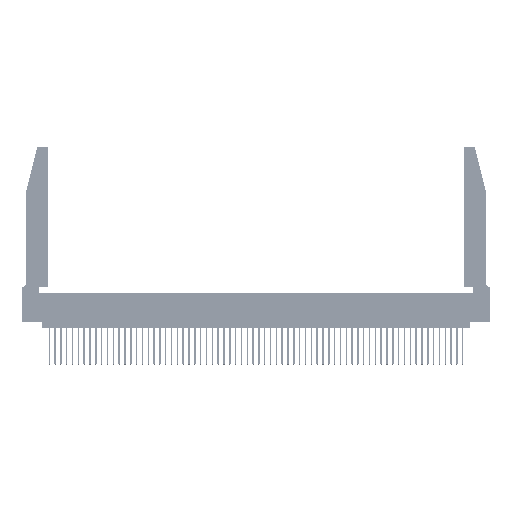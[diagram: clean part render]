
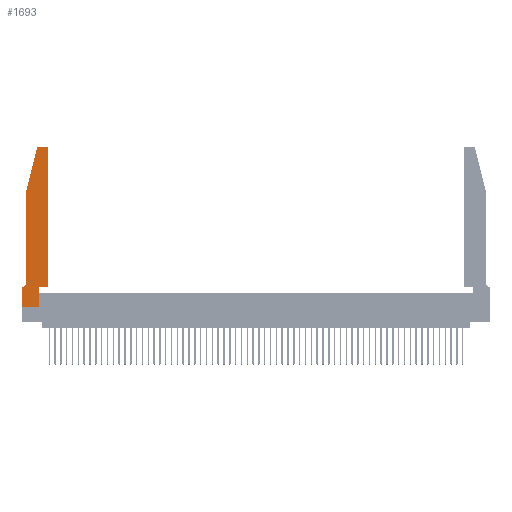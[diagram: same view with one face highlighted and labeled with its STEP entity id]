
A CAD part, top view. The second image highlights one B-rep face of the part: STEP entity #1693.
In plain terms, the highlighted planar face has unit normal (0, 0, 1).
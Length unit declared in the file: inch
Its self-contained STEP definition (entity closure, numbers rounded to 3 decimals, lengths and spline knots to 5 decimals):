
#1656 = CARTESIAN_POINT ( 'NONE',  ( 0.4505, 0.35, 0.37 ) ) ;
#1693 = ADVANCED_FACE ( 'NONE', ( #45413 ), #8325, .T. ) ;
#1998 = ORIENTED_EDGE ( 'NONE', *, *, #39850, .T. ) ;
#2313 = DIRECTION ( 'NONE',  ( -1., 0., 0. ) ) ;
#2681 = VERTEX_POINT ( 'NONE', #39917 ) ;
#3382 = DIRECTION ( 'NONE',  ( 0., 0., 1. ) ) ;
#3571 = EDGE_CURVE ( 'NONE', #25130, #55235, #18703, .T. ) ;
#3941 = LINE ( 'NONE', #18616, #14277 ) ;
#5013 = DIRECTION ( 'NONE',  ( 0., -1., 0. ) ) ;
#5835 = VECTOR ( 'NONE', #31532, 39.37008 ) ;
#6038 = VECTOR ( 'NONE', #40853, 39.37008 ) ;
#6078 = ORIENTED_EDGE ( 'NONE', *, *, #38653, .T. ) ;
#8318 = VERTEX_POINT ( 'NONE', #18544 ) ;
#8325 = PLANE ( 'NONE',  #57042 ) ;
#9174 = CARTESIAN_POINT ( 'NONE',  ( 0.0755, 0.42, 0.37 ) ) ;
#10579 = AXIS2_PLACEMENT_3D ( 'NONE', #34514, #3382, #38793 ) ;
#10895 = DIRECTION ( 'NONE',  ( 1., 0., 0. ) ) ;
#11281 = CARTESIAN_POINT ( 'NONE',  ( 0.284, 2.75, 0.37 ) ) ;
#11627 = LINE ( 'NONE', #30556, #20619 ) ;
#12865 = LINE ( 'NONE', #41238, #6038 ) ;
#14277 = VECTOR ( 'NONE', #27912, 39.37008 ) ;
#16488 = ORIENTED_EDGE ( 'NONE', *, *, #51522, .T. ) ;
#16531 = VERTEX_POINT ( 'NONE', #9174 ) ;
#17021 = CARTESIAN_POINT ( 'NONE',  ( 0., 0.35, 0.37 ) ) ;
#17188 = ORIENTED_EDGE ( 'NONE', *, *, #3571, .T. ) ;
#17287 = VERTEX_POINT ( 'NONE', #27896 ) ;
#17335 = CARTESIAN_POINT ( 'NONE',  ( 0., 0., 0.37 ) ) ;
#18544 = CARTESIAN_POINT ( 'NONE',  ( 0., 0.35, 0.37 ) ) ;
#18616 = CARTESIAN_POINT ( 'NONE',  ( 0.2865, 0.35, 0.37 ) ) ;
#18703 = CIRCLE ( 'NONE', #56364, 0.03 ) ;
#20619 = VECTOR ( 'NONE', #39122, 39.37008 ) ;
#22130 = VERTEX_POINT ( 'NONE', #38931 ) ;
#22216 = CARTESIAN_POINT ( 'NONE',  ( 0.4505, 0.35, 0.37 ) ) ;
#22503 = DIRECTION ( 'NONE',  ( -1., 0., 0. ) ) ;
#23023 = VERTEX_POINT ( 'NONE', #17335 ) ;
#23167 = CARTESIAN_POINT ( 'NONE',  ( 0.0755, 2., 0.37 ) ) ;
#23228 = CARTESIAN_POINT ( 'NONE',  ( 0.25487, 2.72718, 0.37 ) ) ;
#23265 = ORIENTED_EDGE ( 'NONE', *, *, #55868, .T. ) ;
#23733 = LINE ( 'NONE', #31285, #51468 ) ;
#24746 = CARTESIAN_POINT ( 'NONE',  ( 0.0055, 0.35, 0.37 ) ) ;
#24871 = CARTESIAN_POINT ( 'NONE',  ( 0.4505, 0.35, 0.37 ) ) ;
#25130 = VERTEX_POINT ( 'NONE', #11281 ) ;
#25391 = CIRCLE ( 'NONE', #10579, 0.03 ) ;
#26626 = DIRECTION ( 'NONE',  ( 0., -1., 0. ) ) ;
#26824 = CARTESIAN_POINT ( 'NONE',  ( 0., 0., 0.37 ) ) ;
#27221 = LINE ( 'NONE', #53321, #5835 ) ;
#27896 = CARTESIAN_POINT ( 'NONE',  ( 0.2865, 0.35, 0.37 ) ) ;
#27912 = DIRECTION ( 'NONE',  ( 0., 1., 0. ) ) ;
#27951 = EDGE_CURVE ( 'NONE', #49657, #16531, #23733, .T. ) ;
#28055 = CARTESIAN_POINT ( 'NONE',  ( 0.2865, 0., 0.37 ) ) ;
#29270 = EDGE_LOOP ( 'NONE', ( #23265, #17188, #54557, #50282, #1998, #47349, #16488, #56814, #45931, #6078, #56794, #52931 ) ) ;
#29696 = VERTEX_POINT ( 'NONE', #22216 ) ;
#30556 = CARTESIAN_POINT ( 'NONE',  ( 0.0755, 2., 0.37 ) ) ;
#31285 = CARTESIAN_POINT ( 'NONE',  ( 0.0755, 2., 0.37 ) ) ;
#31532 = DIRECTION ( 'NONE',  ( 1., 0., 0. ) ) ;
#31607 = CARTESIAN_POINT ( 'NONE',  ( 0.0755, 0.35, 0.37 ) ) ;
#32679 = CIRCLE ( 'NONE', #56281, 0.07 ) ;
#34514 = CARTESIAN_POINT ( 'NONE',  ( 0.4205, 2.72, 0.37 ) ) ;
#35777 = EDGE_CURVE ( 'NONE', #55235, #49657, #11627, .T. ) ;
#36547 = LINE ( 'NONE', #26824, #56707 ) ;
#36707 = EDGE_CURVE ( 'NONE', #39208, #17287, #3941, .T. ) ;
#37719 = VECTOR ( 'NONE', #10895, 39.37008 ) ;
#37913 = DIRECTION ( 'NONE',  ( 0., 0., -1. ) ) ;
#38653 = EDGE_CURVE ( 'NONE', #17287, #29696, #52315, .T. ) ;
#38656 = DIRECTION ( 'NONE',  ( 1., 0., 0. ) ) ;
#38793 = DIRECTION ( 'NONE',  ( 1., 0., 0. ) ) ;
#38931 = CARTESIAN_POINT ( 'NONE',  ( 0.4505, 2.72, 0.37 ) ) ;
#38968 = EDGE_CURVE ( 'NONE', #23023, #39208, #27221, .T. ) ;
#39122 = DIRECTION ( 'NONE',  ( -0.239, -0.971, 0. ) ) ;
#39125 = DIRECTION ( 'NONE',  ( 0., 0., 1. ) ) ;
#39208 = VERTEX_POINT ( 'NONE', #28055 ) ;
#39850 = EDGE_CURVE ( 'NONE', #16531, #51214, #32679, .T. ) ;
#39917 = CARTESIAN_POINT ( 'NONE',  ( 0.4205, 2.75, 0.37 ) ) ;
#40853 = DIRECTION ( 'NONE',  ( -1., 0., 0. ) ) ;
#41238 = CARTESIAN_POINT ( 'NONE',  ( 0.2605, 2.75, 0.37 ) ) ;
#42366 = CARTESIAN_POINT ( 'NONE',  ( 0.0055, 0.42, 0.37 ) ) ;
#42463 = EDGE_CURVE ( 'NONE', #29696, #22130, #46968, .T. ) ;
#42731 = CARTESIAN_POINT ( 'NONE',  ( 0.284, 2.72, 0.37 ) ) ;
#45413 = FACE_OUTER_BOUND ( 'NONE', #29270, .T. ) ;
#45931 = ORIENTED_EDGE ( 'NONE', *, *, #36707, .T. ) ;
#46968 = LINE ( 'NONE', #24871, #55336 ) ;
#47349 = ORIENTED_EDGE ( 'NONE', *, *, #47984, .T. ) ;
#47984 = EDGE_CURVE ( 'NONE', #51214, #8318, #51271, .T. ) ;
#49657 = VERTEX_POINT ( 'NONE', #23167 ) ;
#50282 = ORIENTED_EDGE ( 'NONE', *, *, #27951, .T. ) ;
#51214 = VERTEX_POINT ( 'NONE', #24746 ) ;
#51271 = LINE ( 'NONE', #31607, #54739 ) ;
#51468 = VECTOR ( 'NONE', #5013, 39.37008 ) ;
#51522 = EDGE_CURVE ( 'NONE', #8318, #23023, #36547, .T. ) ;
#52013 = EDGE_CURVE ( 'NONE', #22130, #2681, #25391, .T. ) ;
#52315 = LINE ( 'NONE', #1656, #37719 ) ;
#52931 = ORIENTED_EDGE ( 'NONE', *, *, #52013, .T. ) ;
#53321 = CARTESIAN_POINT ( 'NONE',  ( 0., 0., 0.37 ) ) ;
#54557 = ORIENTED_EDGE ( 'NONE', *, *, #35777, .T. ) ;
#54739 = VECTOR ( 'NONE', #22503, 39.37008 ) ;
#55235 = VERTEX_POINT ( 'NONE', #23228 ) ;
#55336 = VECTOR ( 'NONE', #55967, 39.37008 ) ;
#55868 = EDGE_CURVE ( 'NONE', #2681, #25130, #12865, .T. ) ;
#55967 = DIRECTION ( 'NONE',  ( 0., 1., 0. ) ) ;
#56281 = AXIS2_PLACEMENT_3D ( 'NONE', #42366, #37913, #2313 ) ;
#56364 = AXIS2_PLACEMENT_3D ( 'NONE', #42731, #56899, #38656 ) ;
#56707 = VECTOR ( 'NONE', #26626, 39.37008 ) ;
#56794 = ORIENTED_EDGE ( 'NONE', *, *, #42463, .T. ) ;
#56814 = ORIENTED_EDGE ( 'NONE', *, *, #38968, .T. ) ;
#56899 = DIRECTION ( 'NONE',  ( 0., 0., 1. ) ) ;
#57042 = AXIS2_PLACEMENT_3D ( 'NONE', #17021, #39125, #57187 ) ;
#57187 = DIRECTION ( 'NONE',  ( 1., 0., 0. ) ) ;
